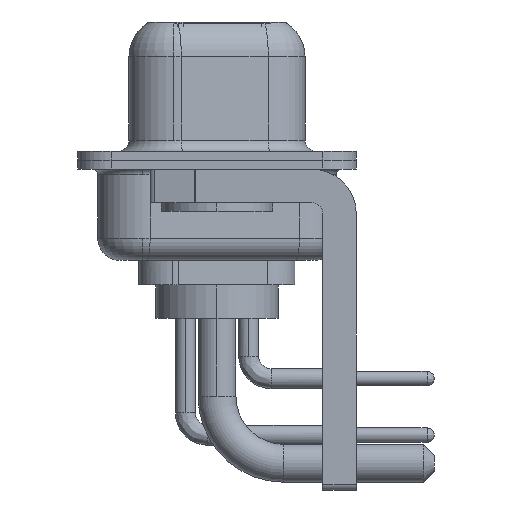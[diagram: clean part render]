
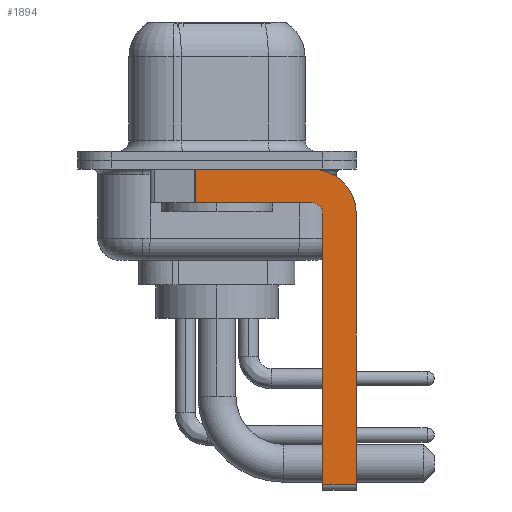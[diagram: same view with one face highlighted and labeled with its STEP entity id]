
A CAD part, left-side view. The second image highlights one B-rep face of the part: STEP entity #1894.
In plain terms, the highlighted planar face has unit normal (-1, 0, 0).
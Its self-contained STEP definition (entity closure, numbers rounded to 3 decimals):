
#835 = CARTESIAN_POINT ( 'NONE',  ( -2.9, -4.25, -2.4 ) ) ;
#1532 = ORIENTED_EDGE ( 'NONE', *, *, #5860, .T. ) ;
#1541 = ORIENTED_EDGE ( 'NONE', *, *, #4570, .T. ) ;
#1894 = ADVANCED_FACE ( 'NONE', ( #15415 ), #6961, .F. ) ;
#2062 = CARTESIAN_POINT ( 'NONE',  ( -2.9, 3., -0.4 ) ) ;
#2489 = DIRECTION ( 'NONE',  ( 0., 0., -1. ) ) ;
#2583 = DIRECTION ( 'NONE',  ( 1., 0., 0. ) ) ;
#2996 = ORIENTED_EDGE ( 'NONE', *, *, #14657, .F. ) ;
#3156 = DIRECTION ( 'NONE',  ( 0., -1., 0. ) ) ;
#3389 = EDGE_CURVE ( 'NONE', #16524, #10687, #6245, .T. ) ;
#3426 = VERTEX_POINT ( 'NONE', #6331 ) ;
#3616 = VECTOR ( 'NONE', #6574, 1000. ) ;
#3765 = EDGE_CURVE ( 'NONE', #10687, #15961, #16023, .T. ) ;
#4108 = EDGE_LOOP ( 'NONE', ( #6004, #1532, #8001, #2996, #13926, #1541, #17495, #15016 ) ) ;
#4335 = DIRECTION ( 'NONE',  ( 0., 0., 1. ) ) ;
#4570 = EDGE_CURVE ( 'NONE', #3426, #15961, #7456, .T. ) ;
#4666 = CARTESIAN_POINT ( 'NONE',  ( -2.9, -6.25, -2.4 ) ) ;
#4801 = LINE ( 'NONE', #2062, #16393 ) ;
#5035 = AXIS2_PLACEMENT_3D ( 'NONE', #835, #13233, #2489 ) ;
#5383 = VECTOR ( 'NONE', #3156, 1000. ) ;
#5516 = CARTESIAN_POINT ( 'NONE',  ( -2.9, -4.25, -0.4 ) ) ;
#5594 = CARTESIAN_POINT ( 'NONE',  ( -2.9, -4.25, -2.4 ) ) ;
#5632 = CARTESIAN_POINT ( 'NONE',  ( -2.9, 0.978, -0.4 ) ) ;
#5860 = EDGE_CURVE ( 'NONE', #5869, #6385, #8388, .T. ) ;
#5869 = VERTEX_POINT ( 'NONE', #5632 ) ;
#5999 = DIRECTION ( 'NONE',  ( 0., 1., 0. ) ) ;
#6004 = ORIENTED_EDGE ( 'NONE', *, *, #6234, .F. ) ;
#6234 = EDGE_CURVE ( 'NONE', #5869, #16524, #4801, .T. ) ;
#6245 = CIRCLE ( 'NONE', #5035, 2. ) ;
#6331 = CARTESIAN_POINT ( 'NONE',  ( -2.9, -4.75, -14.55 ) ) ;
#6385 = VERTEX_POINT ( 'NONE', #17893 ) ;
#6574 = DIRECTION ( 'NONE',  ( 0., 0., -1. ) ) ;
#6961 = PLANE ( 'NONE',  #18017 ) ;
#7456 = LINE ( 'NONE', #9903, #5383 ) ;
#7834 = CARTESIAN_POINT ( 'NONE',  ( -2.9, -6.25, -14.55 ) ) ;
#8001 = ORIENTED_EDGE ( 'NONE', *, *, #8467, .F. ) ;
#8163 = DIRECTION ( 'NONE',  ( 0., 0., -1. ) ) ;
#8388 = LINE ( 'NONE', #17914, #16029 ) ;
#8467 = EDGE_CURVE ( 'NONE', #17046, #6385, #11375, .T. ) ;
#8476 = CARTESIAN_POINT ( 'NONE',  ( -2.9, -4.75, -2.4 ) ) ;
#8749 = LINE ( 'NONE', #13341, #13757 ) ;
#9732 = DIRECTION ( 'NONE',  ( 0., 0., -1. ) ) ;
#9903 = CARTESIAN_POINT ( 'NONE',  ( -2.9, -4.25, -14.55 ) ) ;
#10687 = VERTEX_POINT ( 'NONE', #4666 ) ;
#11174 = AXIS2_PLACEMENT_3D ( 'NONE', #16796, #16711, #4335 ) ;
#11375 = LINE ( 'NONE', #15642, #17715 ) ;
#12118 = CARTESIAN_POINT ( 'NONE',  ( -2.9, -6.25, -2.4 ) ) ;
#12842 = EDGE_CURVE ( 'NONE', #3426, #17697, #8749, .T. ) ;
#13233 = DIRECTION ( 'NONE',  ( 1., 0., 0. ) ) ;
#13263 = DIRECTION ( 'NONE',  ( 0., -1., 0. ) ) ;
#13341 = CARTESIAN_POINT ( 'NONE',  ( -2.9, -4.75, -14.8 ) ) ;
#13757 = VECTOR ( 'NONE', #16912, 1000. ) ;
#13926 = ORIENTED_EDGE ( 'NONE', *, *, #12842, .F. ) ;
#14657 = EDGE_CURVE ( 'NONE', #17697, #17046, #16676, .T. ) ;
#15016 = ORIENTED_EDGE ( 'NONE', *, *, #3389, .F. ) ;
#15406 = CARTESIAN_POINT ( 'NONE',  ( -2.9, -4.25, -1.9 ) ) ;
#15415 = FACE_OUTER_BOUND ( 'NONE', #4108, .T. ) ;
#15642 = CARTESIAN_POINT ( 'NONE',  ( -2.9, -4.25, -1.9 ) ) ;
#15961 = VERTEX_POINT ( 'NONE', #7834 ) ;
#16023 = LINE ( 'NONE', #12118, #3616 ) ;
#16029 = VECTOR ( 'NONE', #9732, 1000. ) ;
#16393 = VECTOR ( 'NONE', #13263, 1000. ) ;
#16524 = VERTEX_POINT ( 'NONE', #5516 ) ;
#16676 = CIRCLE ( 'NONE', #11174, 0.5 ) ;
#16711 = DIRECTION ( 'NONE',  ( -1., 0., 0. ) ) ;
#16796 = CARTESIAN_POINT ( 'NONE',  ( -2.9, -4.25, -2.4 ) ) ;
#16912 = DIRECTION ( 'NONE',  ( 0., 0., 1. ) ) ;
#17046 = VERTEX_POINT ( 'NONE', #15406 ) ;
#17495 = ORIENTED_EDGE ( 'NONE', *, *, #3765, .F. ) ;
#17697 = VERTEX_POINT ( 'NONE', #8476 ) ;
#17715 = VECTOR ( 'NONE', #5999, 1000. ) ;
#17893 = CARTESIAN_POINT ( 'NONE',  ( -2.9, 0.978, -1.9 ) ) ;
#17914 = CARTESIAN_POINT ( 'NONE',  ( -2.9, 0.978, -1.9 ) ) ;
#18017 = AXIS2_PLACEMENT_3D ( 'NONE', #5594, #2583, #8163 ) ;
